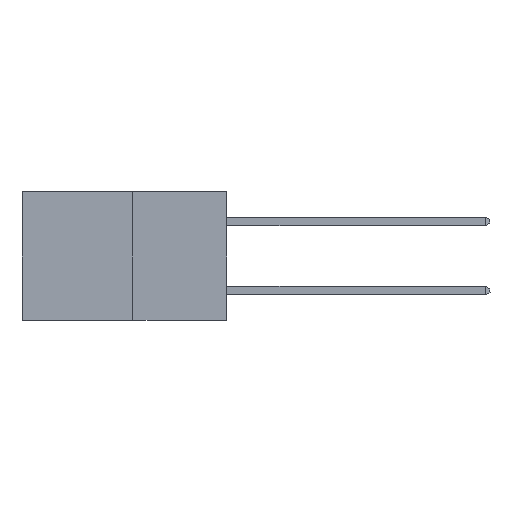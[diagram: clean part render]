
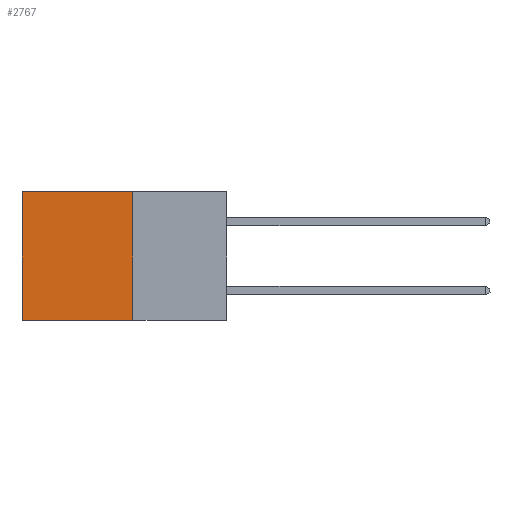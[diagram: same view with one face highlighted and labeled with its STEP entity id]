
A CAD part, left-side view. The second image highlights one B-rep face of the part: STEP entity #2767.
In plain terms, the highlighted planar face has unit normal (-1, 0, 0).
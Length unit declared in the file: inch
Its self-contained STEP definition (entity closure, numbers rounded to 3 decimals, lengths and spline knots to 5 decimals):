
#1914 = DIRECTION ( 'NONE',  ( 0., 0., -1. ) ) ;
#2121 = ORIENTED_EDGE ( 'NONE', *, *, #25610, .T. ) ;
#2392 = DIRECTION ( 'NONE',  ( 0., 0., -1. ) ) ;
#2767 = ADVANCED_FACE ( 'NONE', ( #16493 ), #22455, .F. ) ;
#4768 = DIRECTION ( 'NONE',  ( 0., 1., 0. ) ) ;
#4914 = CARTESIAN_POINT ( 'NONE',  ( 0.277, 0.59, -0.37 ) ) ;
#5308 = AXIS2_PLACEMENT_3D ( 'NONE', #10170, #5995, #20344 ) ;
#5995 = DIRECTION ( 'NONE',  ( 1., 0., 0. ) ) ;
#7148 = CARTESIAN_POINT ( 'NONE',  ( 0.277, 0.27, 0. ) ) ;
#7894 = EDGE_CURVE ( 'NONE', #30186, #15451, #9335, .T. ) ;
#9335 = LINE ( 'NONE', #15409, #27839 ) ;
#10170 = CARTESIAN_POINT ( 'NONE',  ( 0.277, 0.27, -0.37 ) ) ;
#11284 = ORIENTED_EDGE ( 'NONE', *, *, #7894, .F. ) ;
#11751 = EDGE_CURVE ( 'NONE', #13364, #15451, #22037, .T. ) ;
#12000 = CARTESIAN_POINT ( 'NONE',  ( 0.277, 0.27, 0. ) ) ;
#12232 = LINE ( 'NONE', #14533, #30642 ) ;
#12982 = DIRECTION ( 'NONE',  ( 0., 1., 0. ) ) ;
#13364 = VERTEX_POINT ( 'NONE', #21413 ) ;
#14533 = CARTESIAN_POINT ( 'NONE',  ( 0.277, 0.27, -0.37 ) ) ;
#15409 = CARTESIAN_POINT ( 'NONE',  ( 0.277, 0.27, -0.37 ) ) ;
#15451 = VERTEX_POINT ( 'NONE', #4914 ) ;
#15664 = VECTOR ( 'NONE', #4768, 39.37008 ) ;
#16493 = FACE_OUTER_BOUND ( 'NONE', #16972, .T. ) ;
#16972 = EDGE_LOOP ( 'NONE', ( #31095, #11284, #25365, #2121 ) ) ;
#19226 = CARTESIAN_POINT ( 'NONE',  ( 0.277, 0.27, -0.37 ) ) ;
#19446 = LINE ( 'NONE', #7148, #15664 ) ;
#20344 = DIRECTION ( 'NONE',  ( 0., 0., -1. ) ) ;
#21413 = CARTESIAN_POINT ( 'NONE',  ( 0.277, 0.59, 0. ) ) ;
#22037 = LINE ( 'NONE', #30937, #27643 ) ;
#22455 = PLANE ( 'NONE',  #5308 ) ;
#25365 = ORIENTED_EDGE ( 'NONE', *, *, #25632, .F. ) ;
#25610 = EDGE_CURVE ( 'NONE', #30221, #13364, #19446, .T. ) ;
#25632 = EDGE_CURVE ( 'NONE', #30221, #30186, #12232, .T. ) ;
#27643 = VECTOR ( 'NONE', #1914, 39.37008 ) ;
#27839 = VECTOR ( 'NONE', #12982, 39.37008 ) ;
#30186 = VERTEX_POINT ( 'NONE', #19226 ) ;
#30221 = VERTEX_POINT ( 'NONE', #12000 ) ;
#30642 = VECTOR ( 'NONE', #2392, 39.37008 ) ;
#30937 = CARTESIAN_POINT ( 'NONE',  ( 0.277, 0.59, -0.37 ) ) ;
#31095 = ORIENTED_EDGE ( 'NONE', *, *, #11751, .T. ) ;
